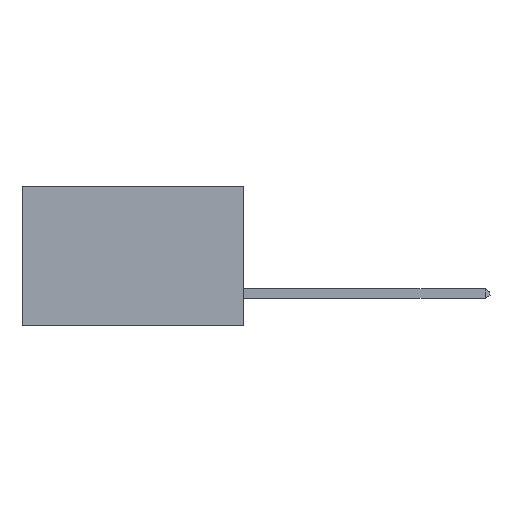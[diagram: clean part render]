
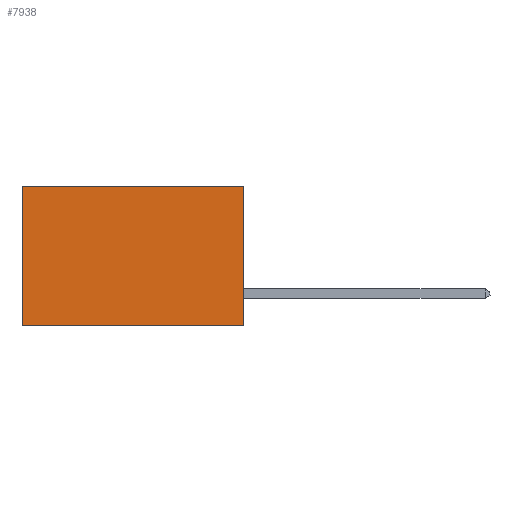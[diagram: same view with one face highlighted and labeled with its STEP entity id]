
A CAD part, left-side view. The second image highlights one B-rep face of the part: STEP entity #7938.
In plain terms, the highlighted planar face has unit normal (-1, 0, 0).
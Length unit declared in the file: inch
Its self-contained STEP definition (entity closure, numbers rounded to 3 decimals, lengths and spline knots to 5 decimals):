
#673 = VERTEX_POINT ( 'NONE', #4921 ) ;
#1149 = VERTEX_POINT ( 'NONE', #6537 ) ;
#1311 = EDGE_CURVE ( 'NONE', #673, #10175, #2868, .T. ) ;
#1348 = EDGE_CURVE ( 'NONE', #1149, #673, #1880, .T. ) ;
#1444 = PLANE ( 'NONE',  #10791 ) ;
#1880 = LINE ( 'NONE', #3407, #12025 ) ;
#2168 = VERTEX_POINT ( 'NONE', #5942 ) ;
#2492 = DIRECTION ( 'NONE',  ( 1., 0., 0. ) ) ;
#2519 = VECTOR ( 'NONE', #10841, 39.37008 ) ;
#2535 = CARTESIAN_POINT ( 'NONE',  ( 0.277, 0., 0. ) ) ;
#2719 = CARTESIAN_POINT ( 'NONE',  ( 0.277, 0.59, -0.37 ) ) ;
#2752 = DIRECTION ( 'NONE',  ( 0., 0., -1. ) ) ;
#2868 = LINE ( 'NONE', #4456, #2519 ) ;
#3164 = EDGE_CURVE ( 'NONE', #2168, #10175, #9869, .T. ) ;
#3407 = CARTESIAN_POINT ( 'NONE',  ( 0.277, 0., -0.37 ) ) ;
#3822 = DIRECTION ( 'NONE',  ( 0., 1., 0. ) ) ;
#4456 = CARTESIAN_POINT ( 'NONE',  ( 0.277, 0., -0.37 ) ) ;
#4536 = ORIENTED_EDGE ( 'NONE', *, *, #4550, .T. ) ;
#4550 = EDGE_CURVE ( 'NONE', #1149, #2168, #7008, .T. ) ;
#4921 = CARTESIAN_POINT ( 'NONE',  ( 0.277, 0., -0.37 ) ) ;
#5090 = FACE_OUTER_BOUND ( 'NONE', #5453, .T. ) ;
#5453 = EDGE_LOOP ( 'NONE', ( #11284, #6863, #11541, #4536 ) ) ;
#5942 = CARTESIAN_POINT ( 'NONE',  ( 0.277, 0.59, 0. ) ) ;
#6537 = CARTESIAN_POINT ( 'NONE',  ( 0.277, 0., 0. ) ) ;
#6723 = VECTOR ( 'NONE', #3822, 39.37008 ) ;
#6863 = ORIENTED_EDGE ( 'NONE', *, *, #1311, .F. ) ;
#7008 = LINE ( 'NONE', #2535, #6723 ) ;
#7530 = VECTOR ( 'NONE', #2752, 39.37008 ) ;
#7938 = ADVANCED_FACE ( 'NONE', ( #5090 ), #1444, .F. ) ;
#8515 = CARTESIAN_POINT ( 'NONE',  ( 0.277, 0., -0.37 ) ) ;
#9396 = DIRECTION ( 'NONE',  ( 0., 0., -1. ) ) ;
#9869 = LINE ( 'NONE', #2719, #7530 ) ;
#10175 = VERTEX_POINT ( 'NONE', #10638 ) ;
#10638 = CARTESIAN_POINT ( 'NONE',  ( 0.277, 0.59, -0.37 ) ) ;
#10791 = AXIS2_PLACEMENT_3D ( 'NONE', #8515, #2492, #9396 ) ;
#10841 = DIRECTION ( 'NONE',  ( 0., 1., 0. ) ) ;
#11251 = DIRECTION ( 'NONE',  ( 0., 0., -1. ) ) ;
#11284 = ORIENTED_EDGE ( 'NONE', *, *, #3164, .T. ) ;
#11541 = ORIENTED_EDGE ( 'NONE', *, *, #1348, .F. ) ;
#12025 = VECTOR ( 'NONE', #11251, 39.37008 ) ;
